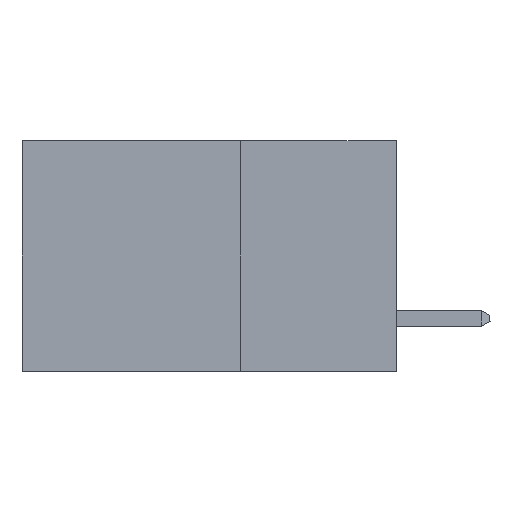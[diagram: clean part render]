
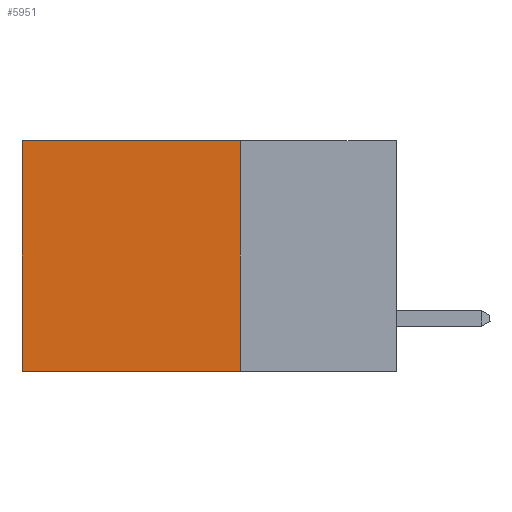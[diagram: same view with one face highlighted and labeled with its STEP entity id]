
A CAD part, left-side view. The second image highlights one B-rep face of the part: STEP entity #5951.
In plain terms, the highlighted planar face has unit normal (-1, 0, 0).
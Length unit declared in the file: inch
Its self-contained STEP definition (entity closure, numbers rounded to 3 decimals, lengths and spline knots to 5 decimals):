
#633 = ORIENTED_EDGE ( 'NONE', *, *, #19732, .F. ) ;
#1283 = LINE ( 'NONE', #18578, #9104 ) ;
#1324 = VECTOR ( 'NONE', #6775, 39.37008 ) ;
#1466 = PLANE ( 'NONE',  #8742 ) ;
#1708 = CARTESIAN_POINT ( 'NONE',  ( 0.298, 0.25, 0. ) ) ;
#1745 = CARTESIAN_POINT ( 'NONE',  ( 0.298, 0.25, -0.37 ) ) ;
#1801 = LINE ( 'NONE', #14483, #1324 ) ;
#2148 = FACE_OUTER_BOUND ( 'NONE', #19250, .T. ) ;
#2695 = DIRECTION ( 'NONE',  ( 0., 1., 0. ) ) ;
#3138 = DIRECTION ( 'NONE',  ( 0., 1., 0. ) ) ;
#3286 = VECTOR ( 'NONE', #2695, 39.37008 ) ;
#3296 = LINE ( 'NONE', #4657, #18434 ) ;
#4657 = CARTESIAN_POINT ( 'NONE',  ( 0.298, 0.25, 0. ) ) ;
#4755 = VERTEX_POINT ( 'NONE', #17516 ) ;
#5951 = ADVANCED_FACE ( 'NONE', ( #2148 ), #1466, .F. ) ;
#6140 = ORIENTED_EDGE ( 'NONE', *, *, #8406, .T. ) ;
#6202 = CARTESIAN_POINT ( 'NONE',  ( 0.298, 0.25, 0. ) ) ;
#6775 = DIRECTION ( 'NONE',  ( 0., 0., -1. ) ) ;
#7028 = EDGE_CURVE ( 'NONE', #10729, #19235, #3296, .T. ) ;
#7495 = LINE ( 'NONE', #15092, #3286 ) ;
#7763 = DIRECTION ( 'NONE',  ( 0., 0., -1. ) ) ;
#8406 = EDGE_CURVE ( 'NONE', #19235, #4755, #1801, .T. ) ;
#8742 = AXIS2_PLACEMENT_3D ( 'NONE', #6202, #17056, #7763 ) ;
#8940 = VERTEX_POINT ( 'NONE', #1745 ) ;
#9104 = VECTOR ( 'NONE', #17077, 39.37008 ) ;
#10729 = VERTEX_POINT ( 'NONE', #1708 ) ;
#10765 = ORIENTED_EDGE ( 'NONE', *, *, #11010, .F. ) ;
#11010 = EDGE_CURVE ( 'NONE', #8940, #4755, #7495, .T. ) ;
#14483 = CARTESIAN_POINT ( 'NONE',  ( 0.298, 0.6, 0. ) ) ;
#15092 = CARTESIAN_POINT ( 'NONE',  ( 0.298, 0.25, -0.37 ) ) ;
#15654 = CARTESIAN_POINT ( 'NONE',  ( 0.298, 0.6, 0. ) ) ;
#17056 = DIRECTION ( 'NONE',  ( 1., 0., 0. ) ) ;
#17077 = DIRECTION ( 'NONE',  ( 0., 0., -1. ) ) ;
#17516 = CARTESIAN_POINT ( 'NONE',  ( 0.298, 0.6, -0.37 ) ) ;
#18434 = VECTOR ( 'NONE', #3138, 39.37008 ) ;
#18578 = CARTESIAN_POINT ( 'NONE',  ( 0.298, 0.25, 0. ) ) ;
#19235 = VERTEX_POINT ( 'NONE', #15654 ) ;
#19250 = EDGE_LOOP ( 'NONE', ( #6140, #10765, #633, #19402 ) ) ;
#19402 = ORIENTED_EDGE ( 'NONE', *, *, #7028, .T. ) ;
#19732 = EDGE_CURVE ( 'NONE', #10729, #8940, #1283, .T. ) ;
